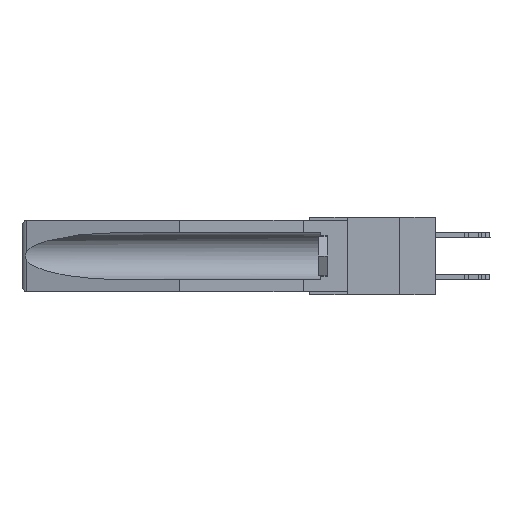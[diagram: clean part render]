
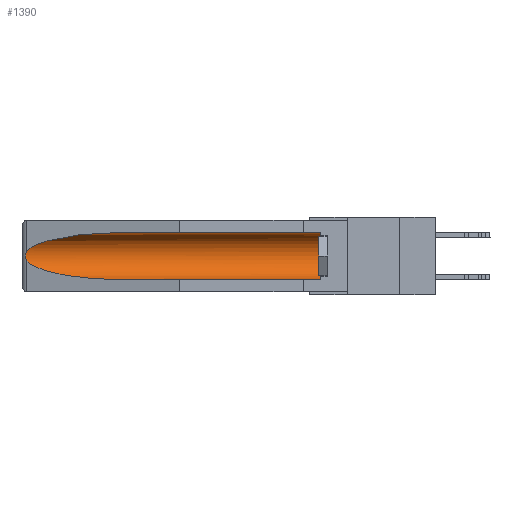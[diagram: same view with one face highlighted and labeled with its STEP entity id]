
A CAD part, left-side view. The second image highlights one B-rep face of the part: STEP entity #1390.
In plain terms, the highlighted cylindrical face has radius 2.857 mm (diameter 5.715 mm), a partial arc.
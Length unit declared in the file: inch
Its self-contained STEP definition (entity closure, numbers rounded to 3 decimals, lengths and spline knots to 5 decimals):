
#313 = CARTESIAN_POINT ( 'NONE',  ( 0.155, 1.07973, -0.059 ) ) ;
#597 = EDGE_CURVE ( 'NONE', #21086, #29514, #6504, .T. ) ;
#1390 = ADVANCED_FACE ( 'NONE', ( #11880 ), #15348, .F. ) ;
#1870 = CARTESIAN_POINT ( 'NONE',  ( 0.155, 1.07973, -0.284 ) ) ;
#1934 = ORIENTED_EDGE ( 'NONE', *, *, #4079, .F. ) ;
#2111 = CARTESIAN_POINT ( 'NONE',  ( 0.26537, 1.52718, -0.19328 ) ) ;
#2556 = ORIENTED_EDGE ( 'NONE', *, *, #17609, .T. ) ;
#3703 =( BOUNDED_CURVE ( )  B_SPLINE_CURVE ( 3, ( #9058, #26328, #31533, #24176 ),
 .UNSPECIFIED., .F., .F. ) 
 B_SPLINE_CURVE_WITH_KNOTS ( ( 4, 4 ),
 ( 0.1948, 1.5708 ),
 .UNSPECIFIED. ) 
 CURVE ( )  GEOMETRIC_REPRESENTATION_ITEM ( )  RATIONAL_B_SPLINE_CURVE ( ( 1., 0.848, 0.848, 1. ) ) 
 REPRESENTATION_ITEM ( '' )  );
#3807 = CARTESIAN_POINT ( 'NONE',  ( 0.155, 0.126, -0.1715 ) ) ;
#3881 = VECTOR ( 'NONE', #25271, 39.37008 ) ;
#4079 = EDGE_CURVE ( 'NONE', #23344, #16851, #11646, .T. ) ;
#4611 = CARTESIAN_POINT ( 'NONE',  ( 0.26537, 1.52718, -0.14972 ) ) ;
#5912 = CARTESIAN_POINT ( 'NONE',  ( 0.155, -0.30754, -0.059 ) ) ;
#6203 = DIRECTION ( 'NONE',  ( 0., -1., 0. ) ) ;
#6504 = B_SPLINE_CURVE_WITH_KNOTS ( 'NONE', 3,
 ( #4611, #16934, #28927, #16714, #23919, #29145, #24021, #26396, #6870, #2111 ),
 .UNSPECIFIED., .F., .F.,
 ( 4, 2, 2, 2, 4 ),
 ( 0., 0.00029, 0.00058, 0.00087, 0.00117 ),
 .UNSPECIFIED. ) ;
#6870 = CARTESIAN_POINT ( 'NONE',  ( 0.26597, 1.5296, -0.19026 ) ) ;
#6936 = DIRECTION ( 'NONE',  ( 0., 1., 0. ) ) ;
#7201 = VERTEX_POINT ( 'NONE', #28769 ) ;
#9058 = CARTESIAN_POINT ( 'NONE',  ( 0.26537, 1.52718, -0.19328 ) ) ;
#11116 = DIRECTION ( 'NONE',  ( 0., 1., 0. ) ) ;
#11646 = LINE ( 'NONE', #15489, #3881 ) ;
#11880 = FACE_OUTER_BOUND ( 'NONE', #12292, .T. ) ;
#12292 = EDGE_LOOP ( 'NONE', ( #17801, #17085, #23910, #1934, #2556, #14383 ) ) ;
#12953 = CARTESIAN_POINT ( 'NONE',  ( 0.26537, 1.52718, -0.14972 ) ) ;
#14383 = ORIENTED_EDGE ( 'NONE', *, *, #17123, .T. ) ;
#14397 = EDGE_CURVE ( 'NONE', #29514, #16851, #3703, .T. ) ;
#15348 = CYLINDRICAL_SURFACE ( 'NONE', #20061, 0.1125 ) ;
#15489 = CARTESIAN_POINT ( 'NONE',  ( 0.155, -0.30754, -0.284 ) ) ;
#16714 = CARTESIAN_POINT ( 'NONE',  ( 0.2673, 1.5327, -0.16383 ) ) ;
#16851 = VERTEX_POINT ( 'NONE', #1870 ) ;
#16934 = CARTESIAN_POINT ( 'NONE',  ( 0.26597, 1.52961, -0.15275 ) ) ;
#16988 = EDGE_CURVE ( 'NONE', #7201, #21086, #29951, .T. ) ;
#17085 = ORIENTED_EDGE ( 'NONE', *, *, #597, .T. ) ;
#17123 = EDGE_CURVE ( 'NONE', #30926, #7201, #18647, .T. ) ;
#17609 = EDGE_CURVE ( 'NONE', #23344, #30926, #20996, .T. ) ;
#17801 = ORIENTED_EDGE ( 'NONE', *, *, #16988, .T. ) ;
#18647 = LINE ( 'NONE', #5912, #24409 ) ;
#19906 = AXIS2_PLACEMENT_3D ( 'NONE', #3807, #6203, #28072 ) ;
#20061 = AXIS2_PLACEMENT_3D ( 'NONE', #21736, #6936, #26664 ) ;
#20996 = CIRCLE ( 'NONE', #19906, 0.1125 ) ;
#21086 = VERTEX_POINT ( 'NONE', #28193 ) ;
#21736 = CARTESIAN_POINT ( 'NONE',  ( 0.155, -0.30754, -0.1715 ) ) ;
#22596 = CARTESIAN_POINT ( 'NONE',  ( 0.155, 0.126, -0.284 ) ) ;
#23344 = VERTEX_POINT ( 'NONE', #22596 ) ;
#23910 = ORIENTED_EDGE ( 'NONE', *, *, #14397, .T. ) ;
#23919 = CARTESIAN_POINT ( 'NONE',  ( 0.2675, 1.53308, -0.16763 ) ) ;
#24021 = CARTESIAN_POINT ( 'NONE',  ( 0.2673, 1.53269, -0.17917 ) ) ;
#24176 = CARTESIAN_POINT ( 'NONE',  ( 0.155, 1.07973, -0.284 ) ) ;
#24409 = VECTOR ( 'NONE', #11116, 39.37008 ) ;
#25220 = CARTESIAN_POINT ( 'NONE',  ( 0.25451, 1.48313, -0.09465 ) ) ;
#25271 = DIRECTION ( 'NONE',  ( 0., 1., 0. ) ) ;
#26328 = CARTESIAN_POINT ( 'NONE',  ( 0.25451, 1.48313, -0.24835 ) ) ;
#26396 = CARTESIAN_POINT ( 'NONE',  ( 0.26655, 1.53094, -0.18657 ) ) ;
#26664 = DIRECTION ( 'NONE',  ( 0., 0., 1. ) ) ;
#27369 = CARTESIAN_POINT ( 'NONE',  ( 0.21114, 1.30732, -0.059 ) ) ;
#28072 = DIRECTION ( 'NONE',  ( 0., 0., 1. ) ) ;
#28193 = CARTESIAN_POINT ( 'NONE',  ( 0.26537, 1.52718, -0.14972 ) ) ;
#28331 = CARTESIAN_POINT ( 'NONE',  ( 0.155, 0.126, -0.059 ) ) ;
#28769 = CARTESIAN_POINT ( 'NONE',  ( 0.155, 1.07973, -0.059 ) ) ;
#28927 = CARTESIAN_POINT ( 'NONE',  ( 0.26654, 1.53092, -0.15636 ) ) ;
#29145 = CARTESIAN_POINT ( 'NONE',  ( 0.2675, 1.53308, -0.17534 ) ) ;
#29446 = CARTESIAN_POINT ( 'NONE',  ( 0.26537, 1.52718, -0.19328 ) ) ;
#29514 = VERTEX_POINT ( 'NONE', #29446 ) ;
#29951 =( BOUNDED_CURVE ( )  B_SPLINE_CURVE ( 3, ( #313, #27369, #25220, #12953 ),
 .UNSPECIFIED., .F., .F. ) 
 B_SPLINE_CURVE_WITH_KNOTS ( ( 4, 4 ),
 ( 4.71239, 6.08839 ),
 .UNSPECIFIED. ) 
 CURVE ( )  GEOMETRIC_REPRESENTATION_ITEM ( )  RATIONAL_B_SPLINE_CURVE ( ( 1., 0.848, 0.848, 1. ) ) 
 REPRESENTATION_ITEM ( '' )  );
#30926 = VERTEX_POINT ( 'NONE', #28331 ) ;
#31533 = CARTESIAN_POINT ( 'NONE',  ( 0.21114, 1.30732, -0.284 ) ) ;
